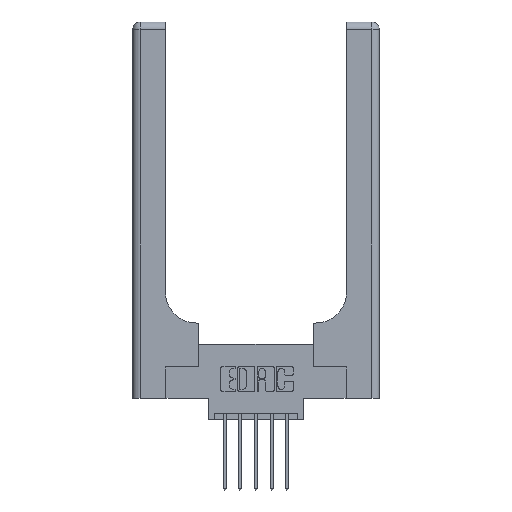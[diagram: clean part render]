
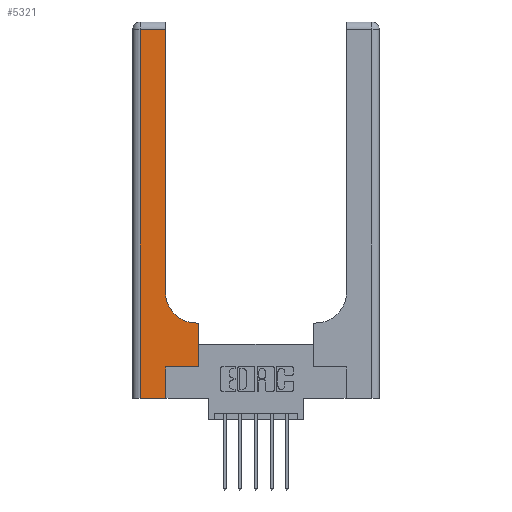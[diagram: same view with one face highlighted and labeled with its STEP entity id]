
A CAD part, top view. The second image highlights one B-rep face of the part: STEP entity #5321.
In plain terms, the highlighted planar face has unit normal (0, 0, 1).
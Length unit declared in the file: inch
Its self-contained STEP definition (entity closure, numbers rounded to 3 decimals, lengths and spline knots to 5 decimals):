
#145 = ORIENTED_EDGE ( 'NONE', *, *, #1034, .T. ) ;
#218 = ORIENTED_EDGE ( 'NONE', *, *, #2759, .T. ) ;
#332 = VERTEX_POINT ( 'NONE', #2943 ) ;
#341 = ORIENTED_EDGE ( 'NONE', *, *, #6960, .T. ) ;
#462 = EDGE_CURVE ( 'NONE', #11935, #11498, #13069, .T. ) ;
#489 = DIRECTION ( 'NONE',  ( 0., -1., 0. ) ) ;
#574 = DIRECTION ( 'NONE',  ( 0., 0., -1. ) ) ;
#591 = CARTESIAN_POINT ( 'NONE',  ( 0.06, 2.94, 0.37 ) ) ;
#644 = EDGE_CURVE ( 'NONE', #1511, #12276, #6313, .T. ) ;
#874 = EDGE_CURVE ( 'NONE', #12276, #10490, #8006, .T. ) ;
#951 = VECTOR ( 'NONE', #7864, 39.37008 ) ;
#994 = CARTESIAN_POINT ( 'NONE',  ( 0.265, 0., 0.37 ) ) ;
#1034 = EDGE_CURVE ( 'NONE', #11498, #3204, #11685, .T. ) ;
#1047 = PLANE ( 'NONE',  #12381 ) ;
#1211 = VECTOR ( 'NONE', #1712, 39.37008 ) ;
#1253 = DIRECTION ( 'NONE',  ( -1., 0., 0. ) ) ;
#1511 = VERTEX_POINT ( 'NONE', #7624 ) ;
#1712 = DIRECTION ( 'NONE',  ( 0., 1., 0. ) ) ;
#1902 = CARTESIAN_POINT ( 'NONE',  ( 0.26, 2.94, 0.37 ) ) ;
#1979 = CARTESIAN_POINT ( 'NONE',  ( 0.265, 0.25, 0.37 ) ) ;
#2468 = CARTESIAN_POINT ( 'NONE',  ( 0., 3., 0.37 ) ) ;
#2759 = EDGE_CURVE ( 'NONE', #10455, #11935, #9062, .T. ) ;
#2879 = DIRECTION ( 'NONE',  ( 0., 1., 0. ) ) ;
#2943 = CARTESIAN_POINT ( 'NONE',  ( 0.51, 0.6, 0.37 ) ) ;
#3204 = VERTEX_POINT ( 'NONE', #4257 ) ;
#3221 = AXIS2_PLACEMENT_3D ( 'NONE', #13401, #574, #4806 ) ;
#3881 = CIRCLE ( 'NONE', #3221, 0.25 ) ;
#4257 = CARTESIAN_POINT ( 'NONE',  ( 0.528, 0.25, 0.37 ) ) ;
#4260 = DIRECTION ( 'NONE',  ( 0., 1., 0. ) ) ;
#4581 = DIRECTION ( 'NONE',  ( -1., 0., 0. ) ) ;
#4806 = DIRECTION ( 'NONE',  ( 1., 0., 0. ) ) ;
#4966 = CARTESIAN_POINT ( 'NONE',  ( 0.06, 0., 0.37 ) ) ;
#5068 = EDGE_CURVE ( 'NONE', #10490, #10455, #7147, .T. ) ;
#5321 = ADVANCED_FACE ( 'NONE', ( #9768 ), #1047, .F. ) ;
#5402 = CARTESIAN_POINT ( 'NONE',  ( 0.265, 0., 0.37 ) ) ;
#5767 = EDGE_LOOP ( 'NONE', ( #8183, #10898, #6686, #218, #10242, #145, #11131, #10280, #341 ) ) ;
#5941 = CARTESIAN_POINT ( 'NONE',  ( 0.26, 0.6, 0.37 ) ) ;
#6061 = EDGE_CURVE ( 'NONE', #3204, #6596, #6265, .T. ) ;
#6265 = LINE ( 'NONE', #9456, #11997 ) ;
#6313 = LINE ( 'NONE', #10638, #1211 ) ;
#6596 = VERTEX_POINT ( 'NONE', #7523 ) ;
#6686 = ORIENTED_EDGE ( 'NONE', *, *, #5068, .T. ) ;
#6960 = EDGE_CURVE ( 'NONE', #332, #1511, #3881, .T. ) ;
#7147 = LINE ( 'NONE', #11270, #12232 ) ;
#7387 = EDGE_CURVE ( 'NONE', #6596, #332, #10137, .T. ) ;
#7523 = CARTESIAN_POINT ( 'NONE',  ( 0.528, 0.6, 0.37 ) ) ;
#7624 = CARTESIAN_POINT ( 'NONE',  ( 0.26, 0.85, 0.37 ) ) ;
#7795 = VECTOR ( 'NONE', #12679, 39.37008 ) ;
#7864 = DIRECTION ( 'NONE',  ( 1., 0., 0. ) ) ;
#8006 = LINE ( 'NONE', #13319, #12323 ) ;
#8183 = ORIENTED_EDGE ( 'NONE', *, *, #644, .T. ) ;
#9062 = LINE ( 'NONE', #13453, #951 ) ;
#9066 = DIRECTION ( 'NONE',  ( -1., 0., 0. ) ) ;
#9456 = CARTESIAN_POINT ( 'NONE',  ( 0.528, 0.25, 0.37 ) ) ;
#9768 = FACE_OUTER_BOUND ( 'NONE', #5767, .T. ) ;
#9909 = DIRECTION ( 'NONE',  ( 0., 0., -1. ) ) ;
#10137 = LINE ( 'NONE', #5941, #10691 ) ;
#10242 = ORIENTED_EDGE ( 'NONE', *, *, #462, .T. ) ;
#10280 = ORIENTED_EDGE ( 'NONE', *, *, #7387, .T. ) ;
#10455 = VERTEX_POINT ( 'NONE', #4966 ) ;
#10490 = VERTEX_POINT ( 'NONE', #591 ) ;
#10638 = CARTESIAN_POINT ( 'NONE',  ( 0.26, 3., 0.37 ) ) ;
#10691 = VECTOR ( 'NONE', #9066, 39.37008 ) ;
#10898 = ORIENTED_EDGE ( 'NONE', *, *, #874, .T. ) ;
#11131 = ORIENTED_EDGE ( 'NONE', *, *, #6061, .T. ) ;
#11270 = CARTESIAN_POINT ( 'NONE',  ( 0.06, 3., 0.37 ) ) ;
#11498 = VERTEX_POINT ( 'NONE', #11938 ) ;
#11685 = LINE ( 'NONE', #1979, #7795 ) ;
#11935 = VERTEX_POINT ( 'NONE', #994 ) ;
#11938 = CARTESIAN_POINT ( 'NONE',  ( 0.265, 0.25, 0.37 ) ) ;
#11997 = VECTOR ( 'NONE', #2879, 39.37008 ) ;
#12232 = VECTOR ( 'NONE', #489, 39.37008 ) ;
#12276 = VERTEX_POINT ( 'NONE', #1902 ) ;
#12323 = VECTOR ( 'NONE', #4581, 39.37008 ) ;
#12381 = AXIS2_PLACEMENT_3D ( 'NONE', #2468, #9909, #1253 ) ;
#12679 = DIRECTION ( 'NONE',  ( 1., 0., 0. ) ) ;
#13069 = LINE ( 'NONE', #5402, #13468 ) ;
#13319 = CARTESIAN_POINT ( 'NONE',  ( 0., 2.94, 0.37 ) ) ;
#13401 = CARTESIAN_POINT ( 'NONE',  ( 0.51, 0.85, 0.37 ) ) ;
#13453 = CARTESIAN_POINT ( 'NONE',  ( 0., 0., 0.37 ) ) ;
#13468 = VECTOR ( 'NONE', #4260, 39.37008 ) ;
